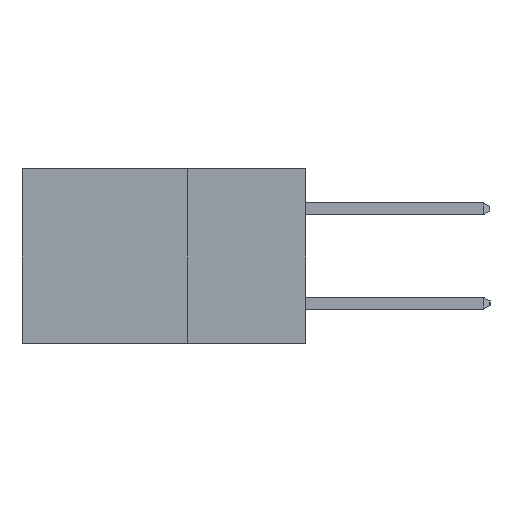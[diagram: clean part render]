
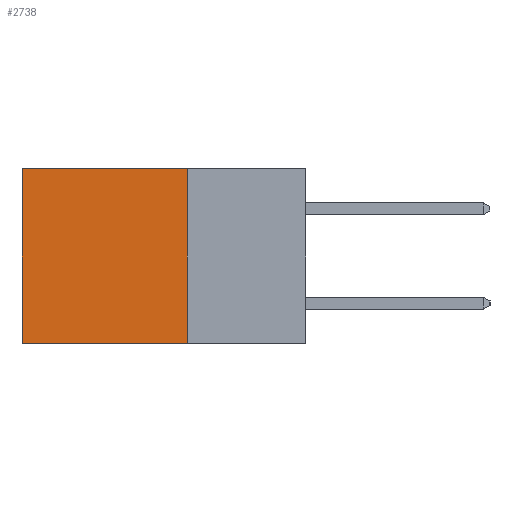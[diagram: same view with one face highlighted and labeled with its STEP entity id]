
A CAD part, left-side view. The second image highlights one B-rep face of the part: STEP entity #2738.
In plain terms, the highlighted planar face has unit normal (-1, 0, 0).
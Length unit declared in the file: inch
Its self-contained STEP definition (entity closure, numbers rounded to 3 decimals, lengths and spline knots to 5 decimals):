
#208 = CARTESIAN_POINT ( 'NONE',  ( 0.2615, 0.6, -0.37 ) ) ;
#209 = DIRECTION ( 'NONE',  ( 1., 0., 0. ) ) ;
#317 = EDGE_LOOP ( 'NONE', ( #5299, #7359, #7627, #9666 ) ) ;
#869 = VECTOR ( 'NONE', #10386, 39.37008 ) ;
#1066 = CARTESIAN_POINT ( 'NONE',  ( 0.2615, 0.25, -0.37 ) ) ;
#1104 = DIRECTION ( 'NONE',  ( 0., 0., -1. ) ) ;
#1106 = DIRECTION ( 'NONE',  ( 0., 1., 0. ) ) ;
#1519 = VECTOR ( 'NONE', #1106, 39.37008 ) ;
#1520 = CARTESIAN_POINT ( 'NONE',  ( 0.2615, 0.25, -0.37 ) ) ;
#2150 = VECTOR ( 'NONE', #7745, 39.37008 ) ;
#2738 = ADVANCED_FACE ( 'NONE', ( #9715 ), #10057, .F. ) ;
#2900 = EDGE_CURVE ( 'NONE', #4656, #7839, #9593, .T. ) ;
#3670 = VECTOR ( 'NONE', #1104, 39.37008 ) ;
#3818 = VERTEX_POINT ( 'NONE', #9789 ) ;
#3877 = LINE ( 'NONE', #4602, #1519 ) ;
#4409 = LINE ( 'NONE', #4586, #2150 ) ;
#4586 = CARTESIAN_POINT ( 'NONE',  ( 0.2615, 0.25, 0. ) ) ;
#4602 = CARTESIAN_POINT ( 'NONE',  ( 0.2615, 0.25, -0.37 ) ) ;
#4656 = VERTEX_POINT ( 'NONE', #8915 ) ;
#5299 = ORIENTED_EDGE ( 'NONE', *, *, #5902, .T. ) ;
#5451 = CARTESIAN_POINT ( 'NONE',  ( 0.2615, 0.25, -0.37 ) ) ;
#5902 = EDGE_CURVE ( 'NONE', #6357, #3818, #9680, .T. ) ;
#6170 = DIRECTION ( 'NONE',  ( 0., 0., -1. ) ) ;
#6357 = VERTEX_POINT ( 'NONE', #7288 ) ;
#6870 = EDGE_CURVE ( 'NONE', #4656, #6357, #4409, .T. ) ;
#7288 = CARTESIAN_POINT ( 'NONE',  ( 0.2615, 0.6, 0. ) ) ;
#7359 = ORIENTED_EDGE ( 'NONE', *, *, #8568, .F. ) ;
#7627 = ORIENTED_EDGE ( 'NONE', *, *, #2900, .F. ) ;
#7745 = DIRECTION ( 'NONE',  ( 0., 1., 0. ) ) ;
#7839 = VERTEX_POINT ( 'NONE', #5451 ) ;
#8568 = EDGE_CURVE ( 'NONE', #7839, #3818, #3877, .T. ) ;
#8915 = CARTESIAN_POINT ( 'NONE',  ( 0.2615, 0.25, 0. ) ) ;
#9479 = AXIS2_PLACEMENT_3D ( 'NONE', #1066, #209, #6170 ) ;
#9593 = LINE ( 'NONE', #1520, #869 ) ;
#9666 = ORIENTED_EDGE ( 'NONE', *, *, #6870, .T. ) ;
#9680 = LINE ( 'NONE', #208, #3670 ) ;
#9715 = FACE_OUTER_BOUND ( 'NONE', #317, .T. ) ;
#9789 = CARTESIAN_POINT ( 'NONE',  ( 0.2615, 0.6, -0.37 ) ) ;
#10057 = PLANE ( 'NONE',  #9479 ) ;
#10386 = DIRECTION ( 'NONE',  ( 0., 0., -1. ) ) ;
